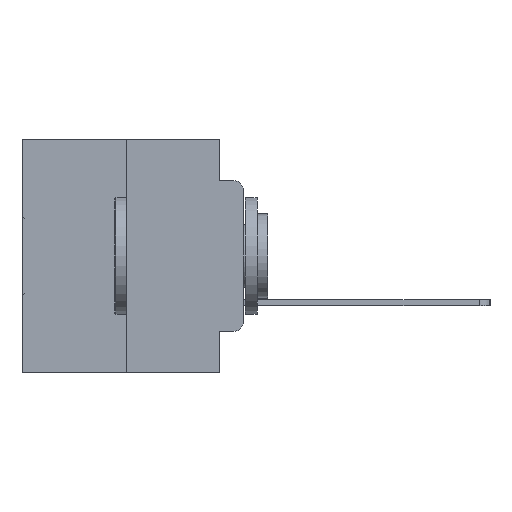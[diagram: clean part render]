
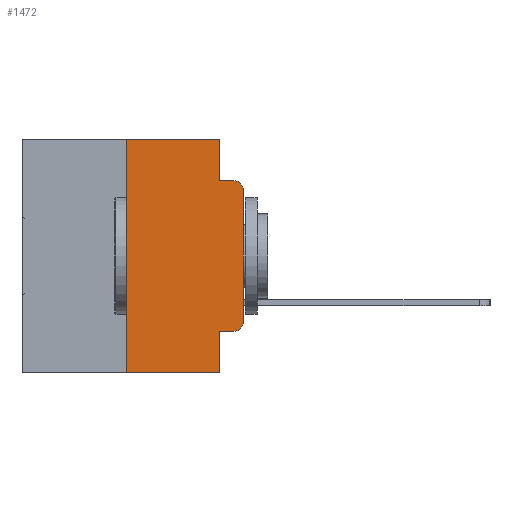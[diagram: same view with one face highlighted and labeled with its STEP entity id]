
A CAD part, left-side view. The second image highlights one B-rep face of the part: STEP entity #1472.
In plain terms, the highlighted planar face has unit normal (-1, 0, 0).
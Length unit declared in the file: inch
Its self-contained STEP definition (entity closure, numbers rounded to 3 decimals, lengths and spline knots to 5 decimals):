
#870 = ORIENTED_EDGE ( 'NONE', *, *, #10974, .T. ) ;
#1320 = LINE ( 'NONE', #20140, #7169 ) ;
#1391 = CARTESIAN_POINT ( 'NONE',  ( 0., 0.25, -0.5 ) ) ;
#1430 = CARTESIAN_POINT ( 'NONE',  ( 0., 0.051, -0.0885 ) ) ;
#1472 = ADVANCED_FACE ( 'NONE', ( #17701 ), #9680, .F. ) ;
#1654 = EDGE_CURVE ( 'NONE', #9826, #2809, #31042, .T. ) ;
#1736 = DIRECTION ( 'NONE',  ( 0., 0., -1. ) ) ;
#1865 = CARTESIAN_POINT ( 'NONE',  ( 0., 0., 0. ) ) ;
#1971 = DIRECTION ( 'NONE',  ( 0., 0., -1. ) ) ;
#2154 = CARTESIAN_POINT ( 'NONE',  ( 0., 0.473, -0.5 ) ) ;
#2809 = VERTEX_POINT ( 'NONE', #29618 ) ;
#3020 = CARTESIAN_POINT ( 'NONE',  ( 0., 0.051, 0. ) ) ;
#3087 = CARTESIAN_POINT ( 'NONE',  ( 0., 0., -0.1085 ) ) ;
#4046 = VERTEX_POINT ( 'NONE', #25034 ) ;
#5310 = VERTEX_POINT ( 'NONE', #3020 ) ;
#5503 = DIRECTION ( 'NONE',  ( 0., -1., 0. ) ) ;
#5567 = CARTESIAN_POINT ( 'NONE',  ( 0., 0.473, 0. ) ) ;
#6462 = EDGE_CURVE ( 'NONE', #28830, #16751, #1320, .T. ) ;
#6668 = VERTEX_POINT ( 'NONE', #1391 ) ;
#7125 = VERTEX_POINT ( 'NONE', #3087 ) ;
#7169 = VECTOR ( 'NONE', #5503, 39.37008 ) ;
#7835 = DIRECTION ( 'NONE',  ( -1., 0., 0. ) ) ;
#7866 = ORIENTED_EDGE ( 'NONE', *, *, #25582, .T. ) ;
#8071 = CIRCLE ( 'NONE', #11039, 0.02 ) ;
#8243 = CIRCLE ( 'NONE', #14318, 0.02 ) ;
#9408 = ORIENTED_EDGE ( 'NONE', *, *, #1654, .F. ) ;
#9647 = DIRECTION ( 'NONE',  ( 0., -1., 0. ) ) ;
#9680 = PLANE ( 'NONE',  #17693 ) ;
#9826 = VERTEX_POINT ( 'NONE', #14761 ) ;
#10861 = EDGE_CURVE ( 'NONE', #16751, #4046, #8071, .T. ) ;
#10974 = EDGE_CURVE ( 'NONE', #6668, #16359, #14080, .T. ) ;
#11039 = AXIS2_PLACEMENT_3D ( 'NONE', #31024, #16427, #1736 ) ;
#11987 = LINE ( 'NONE', #31257, #24186 ) ;
#12435 = ORIENTED_EDGE ( 'NONE', *, *, #26545, .F. ) ;
#12662 = EDGE_CURVE ( 'NONE', #5310, #9826, #28163, .T. ) ;
#12747 = EDGE_LOOP ( 'NONE', ( #12796, #7866, #9408, #28833, #17353, #12435, #870, #20825, #25478, #15518 ) ) ;
#12796 = ORIENTED_EDGE ( 'NONE', *, *, #28685, .T. ) ;
#13326 = VECTOR ( 'NONE', #9647, 39.37008 ) ;
#14080 = LINE ( 'NONE', #2154, #13326 ) ;
#14110 = CARTESIAN_POINT ( 'NONE',  ( 0., 0.02, -0.4115 ) ) ;
#14258 = DIRECTION ( 'NONE',  ( 1., 0., 0. ) ) ;
#14318 = AXIS2_PLACEMENT_3D ( 'NONE', #22419, #7835, #24864 ) ;
#14761 = CARTESIAN_POINT ( 'NONE',  ( 0., 0.051, -0.0885 ) ) ;
#14967 = DIRECTION ( 'NONE',  ( 0., 0., -1. ) ) ;
#15518 = ORIENTED_EDGE ( 'NONE', *, *, #10861, .T. ) ;
#15713 = DIRECTION ( 'NONE',  ( 0., 0., -1. ) ) ;
#16359 = VERTEX_POINT ( 'NONE', #29613 ) ;
#16427 = DIRECTION ( 'NONE',  ( -1., 0., 0. ) ) ;
#16552 = DIRECTION ( 'NONE',  ( 0., 0., 1. ) ) ;
#16656 = EDGE_CURVE ( 'NONE', #19282, #5310, #17980, .T. ) ;
#16751 = VERTEX_POINT ( 'NONE', #14110 ) ;
#17353 = ORIENTED_EDGE ( 'NONE', *, *, #16656, .F. ) ;
#17613 = DIRECTION ( 'NONE',  ( 0., -1., 0. ) ) ;
#17627 = DIRECTION ( 'NONE',  ( 0., 0., 1. ) ) ;
#17693 = AXIS2_PLACEMENT_3D ( 'NONE', #5567, #14258, #14967 ) ;
#17701 = FACE_OUTER_BOUND ( 'NONE', #12747, .T. ) ;
#17980 = LINE ( 'NONE', #28429, #30952 ) ;
#18847 = VECTOR ( 'NONE', #17613, 39.37008 ) ;
#19282 = VERTEX_POINT ( 'NONE', #22650 ) ;
#19630 = CARTESIAN_POINT ( 'NONE',  ( 0., 0.051, -0.4115 ) ) ;
#19965 = VECTOR ( 'NONE', #16552, 39.37008 ) ;
#20140 = CARTESIAN_POINT ( 'NONE',  ( 0., 0.051, -0.4115 ) ) ;
#20825 = ORIENTED_EDGE ( 'NONE', *, *, #28693, .F. ) ;
#22419 = CARTESIAN_POINT ( 'NONE',  ( 0., 0.02, -0.1085 ) ) ;
#22433 = VECTOR ( 'NONE', #15713, 39.37008 ) ;
#22650 = CARTESIAN_POINT ( 'NONE',  ( 0., 0.25, 0. ) ) ;
#24186 = VECTOR ( 'NONE', #1971, 39.37008 ) ;
#24864 = DIRECTION ( 'NONE',  ( 0., 0., -1. ) ) ;
#25034 = CARTESIAN_POINT ( 'NONE',  ( 0., 0., -0.3915 ) ) ;
#25099 = VECTOR ( 'NONE', #17627, 39.37008 ) ;
#25478 = ORIENTED_EDGE ( 'NONE', *, *, #6462, .T. ) ;
#25556 = CARTESIAN_POINT ( 'NONE',  ( 0., 0.051, 0. ) ) ;
#25582 = EDGE_CURVE ( 'NONE', #7125, #2809, #8243, .T. ) ;
#25732 = LINE ( 'NONE', #1865, #19965 ) ;
#26545 = EDGE_CURVE ( 'NONE', #6668, #19282, #31531, .T. ) ;
#27363 = CARTESIAN_POINT ( 'NONE',  ( 0., 0.25, 0. ) ) ;
#28163 = LINE ( 'NONE', #25556, #22433 ) ;
#28429 = CARTESIAN_POINT ( 'NONE',  ( 0., 0.473, 0. ) ) ;
#28685 = EDGE_CURVE ( 'NONE', #4046, #7125, #25732, .T. ) ;
#28693 = EDGE_CURVE ( 'NONE', #28830, #16359, #11987, .T. ) ;
#28830 = VERTEX_POINT ( 'NONE', #19630 ) ;
#28833 = ORIENTED_EDGE ( 'NONE', *, *, #12662, .F. ) ;
#29613 = CARTESIAN_POINT ( 'NONE',  ( 0., 0.051, -0.5 ) ) ;
#29618 = CARTESIAN_POINT ( 'NONE',  ( 0., 0.02, -0.0885 ) ) ;
#30842 = DIRECTION ( 'NONE',  ( 0., -1., 0. ) ) ;
#30952 = VECTOR ( 'NONE', #30842, 39.37008 ) ;
#31024 = CARTESIAN_POINT ( 'NONE',  ( 0., 0.02, -0.3915 ) ) ;
#31042 = LINE ( 'NONE', #1430, #18847 ) ;
#31257 = CARTESIAN_POINT ( 'NONE',  ( 0., 0.051, 0. ) ) ;
#31531 = LINE ( 'NONE', #27363, #25099 ) ;
